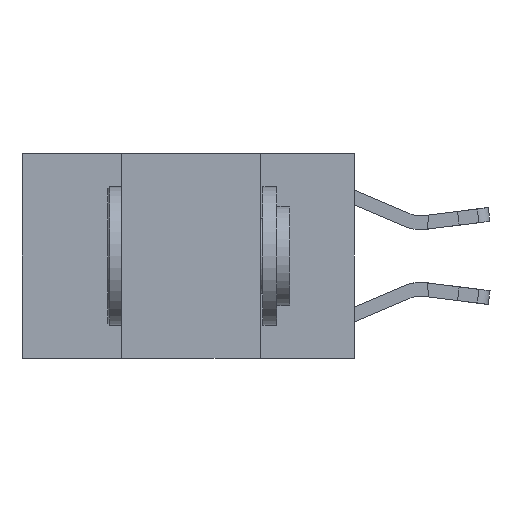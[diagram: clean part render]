
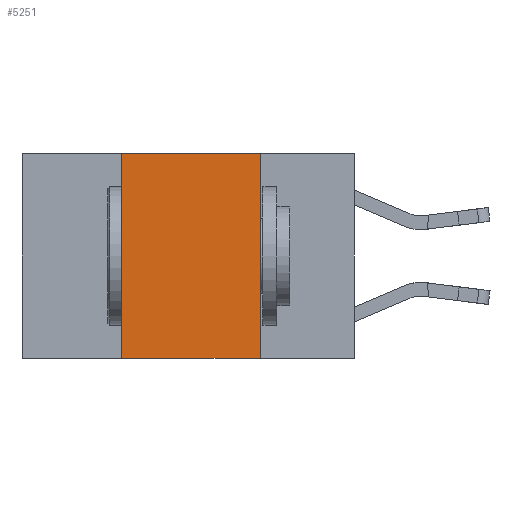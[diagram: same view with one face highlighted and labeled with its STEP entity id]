
A CAD part, left-side view. The second image highlights one B-rep face of the part: STEP entity #5251.
In plain terms, the highlighted planar face has unit normal (-1, 0, 0).
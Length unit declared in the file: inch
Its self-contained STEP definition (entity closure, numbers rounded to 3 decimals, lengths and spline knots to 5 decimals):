
#125 = LINE ( 'NONE', #12262, #6187 ) ;
#1020 = DIRECTION ( 'NONE',  ( 1., 0., 0. ) ) ;
#1275 = CARTESIAN_POINT ( 'NONE',  ( 0., 0.42, 0. ) ) ;
#2204 = EDGE_LOOP ( 'NONE', ( #2734, #13698, #5681, #6448 ) ) ;
#2266 = LINE ( 'NONE', #12846, #5531 ) ;
#2351 = VERTEX_POINT ( 'NONE', #1275 ) ;
#2381 = EDGE_CURVE ( 'NONE', #15526, #12050, #125, .T. ) ;
#2734 = ORIENTED_EDGE ( 'NONE', *, *, #2381, .F. ) ;
#3239 = DIRECTION ( 'NONE',  ( 0., -1., 0. ) ) ;
#3831 = DIRECTION ( 'NONE',  ( 0., 0., -1. ) ) ;
#4308 = LINE ( 'NONE', #8007, #13530 ) ;
#4415 = DIRECTION ( 'NONE',  ( 0., -1., 0. ) ) ;
#4548 = CARTESIAN_POINT ( 'NONE',  ( 0., 0.17, -0.37 ) ) ;
#4798 = VECTOR ( 'NONE', #11339, 39.37008 ) ;
#5051 = EDGE_CURVE ( 'NONE', #14148, #2351, #5177, .T. ) ;
#5177 = LINE ( 'NONE', #5297, #4798 ) ;
#5251 = ADVANCED_FACE ( 'NONE', ( #8537 ), #15459, .F. ) ;
#5297 = CARTESIAN_POINT ( 'NONE',  ( 0., 0.42, 0. ) ) ;
#5531 = VECTOR ( 'NONE', #4415, 39.37008 ) ;
#5681 = ORIENTED_EDGE ( 'NONE', *, *, #5051, .F. ) ;
#6187 = VECTOR ( 'NONE', #3831, 39.37008 ) ;
#6448 = ORIENTED_EDGE ( 'NONE', *, *, #13317, .T. ) ;
#7832 = CARTESIAN_POINT ( 'NONE',  ( 0., 0.42, -0.37 ) ) ;
#8007 = CARTESIAN_POINT ( 'NONE',  ( 0., 0.6, 0. ) ) ;
#8537 = FACE_OUTER_BOUND ( 'NONE', #2204, .T. ) ;
#9503 = DIRECTION ( 'NONE',  ( 0., 0., -1. ) ) ;
#10408 = EDGE_CURVE ( 'NONE', #2351, #15526, #4308, .T. ) ;
#11339 = DIRECTION ( 'NONE',  ( 0., 0., 1. ) ) ;
#12050 = VERTEX_POINT ( 'NONE', #4548 ) ;
#12262 = CARTESIAN_POINT ( 'NONE',  ( 0., 0.17, 0. ) ) ;
#12846 = CARTESIAN_POINT ( 'NONE',  ( 0., 0.6, -0.37 ) ) ;
#13040 = CARTESIAN_POINT ( 'NONE',  ( 0., 0.17, 0. ) ) ;
#13274 = AXIS2_PLACEMENT_3D ( 'NONE', #14293, #1020, #9503 ) ;
#13317 = EDGE_CURVE ( 'NONE', #14148, #12050, #2266, .T. ) ;
#13530 = VECTOR ( 'NONE', #3239, 39.37008 ) ;
#13698 = ORIENTED_EDGE ( 'NONE', *, *, #10408, .F. ) ;
#14148 = VERTEX_POINT ( 'NONE', #7832 ) ;
#14293 = CARTESIAN_POINT ( 'NONE',  ( 0., 0.6, 0. ) ) ;
#15459 = PLANE ( 'NONE',  #13274 ) ;
#15526 = VERTEX_POINT ( 'NONE', #13040 ) ;
